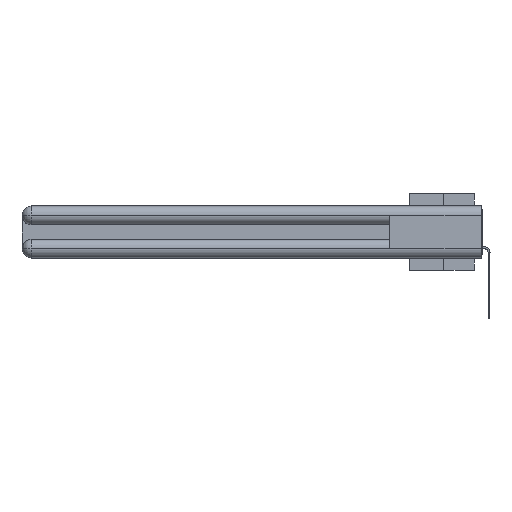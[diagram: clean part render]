
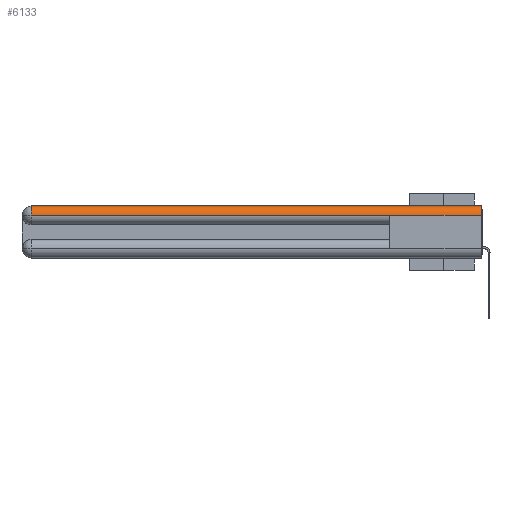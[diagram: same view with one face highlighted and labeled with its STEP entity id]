
A CAD part, left-side view. The second image highlights one B-rep face of the part: STEP entity #6133.
In plain terms, the highlighted cylindrical face has radius 1.562 mm (diameter 3.124 mm), a partial arc.
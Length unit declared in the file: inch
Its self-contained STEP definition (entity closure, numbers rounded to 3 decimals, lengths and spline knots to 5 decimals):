
#640 = VERTEX_POINT ( 'NONE', #28494 ) ;
#670 = VERTEX_POINT ( 'NONE', #4784 ) ;
#1827 = ORIENTED_EDGE ( 'NONE', *, *, #25574, .F. ) ;
#1966 = CARTESIAN_POINT ( 'NONE',  ( 0.0615, 2.94, -0.0615 ) ) ;
#2603 = DIRECTION ( 'NONE',  ( 0., -1., 0. ) ) ;
#3129 = CIRCLE ( 'NONE', #20891, 0.0615 ) ;
#4360 = DIRECTION ( 'NONE',  ( 0., 0., 1. ) ) ;
#4784 = CARTESIAN_POINT ( 'NONE',  ( 0.0615, 0., 0. ) ) ;
#6133 = ADVANCED_FACE ( 'NONE', ( #8679 ), #9038, .T. ) ;
#7046 = VERTEX_POINT ( 'NONE', #27133 ) ;
#7271 = DIRECTION ( 'NONE',  ( 1., 0., 0. ) ) ;
#7306 = DIRECTION ( 'NONE',  ( 0., -1., 0. ) ) ;
#8679 = FACE_OUTER_BOUND ( 'NONE', #14343, .T. ) ;
#9038 = CYLINDRICAL_SURFACE ( 'NONE', #29739, 0.0615 ) ;
#9051 = LINE ( 'NONE', #30841, #21299 ) ;
#9223 = LINE ( 'NONE', #12242, #25432 ) ;
#11766 = DIRECTION ( 'NONE',  ( 0., 1., 0. ) ) ;
#11926 = ORIENTED_EDGE ( 'NONE', *, *, #16208, .T. ) ;
#11950 = EDGE_CURVE ( 'NONE', #670, #27928, #26393, .T. ) ;
#12242 = CARTESIAN_POINT ( 'NONE',  ( 0., 3., -0.0615 ) ) ;
#13227 = EDGE_CURVE ( 'NONE', #27928, #7046, #9223, .T. ) ;
#13975 = DIRECTION ( 'NONE',  ( 0., 0., 1. ) ) ;
#14343 = EDGE_LOOP ( 'NONE', ( #1827, #11926, #28306, #26426, #21880 ) ) ;
#16208 = EDGE_CURVE ( 'NONE', #22157, #640, #3129, .T. ) ;
#16525 = DIRECTION ( 'NONE',  ( 0., 1., 0. ) ) ;
#16729 = VECTOR ( 'NONE', #21988, 39.37008 ) ;
#16813 = CARTESIAN_POINT ( 'NONE',  ( 0.0615, 0., -0.0615 ) ) ;
#17289 = DIRECTION ( 'NONE',  ( 0., -1., 0. ) ) ;
#20286 = AXIS2_PLACEMENT_3D ( 'NONE', #16813, #17289, #7271 ) ;
#20891 = AXIS2_PLACEMENT_3D ( 'NONE', #1966, #2603, #4360 ) ;
#21299 = VECTOR ( 'NONE', #7306, 39.37008 ) ;
#21880 = ORIENTED_EDGE ( 'NONE', *, *, #11950, .F. ) ;
#21988 = DIRECTION ( 'NONE',  ( 0., -1., 0. ) ) ;
#22157 = VERTEX_POINT ( 'NONE', #23263 ) ;
#23263 = CARTESIAN_POINT ( 'NONE',  ( 0.0615, 2.94, 0. ) ) ;
#24323 = CARTESIAN_POINT ( 'NONE',  ( 0., 0., -0.0615 ) ) ;
#24378 = LINE ( 'NONE', #29320, #16729 ) ;
#25432 = VECTOR ( 'NONE', #16525, 39.37008 ) ;
#25574 = EDGE_CURVE ( 'NONE', #22157, #670, #9051, .T. ) ;
#26393 = CIRCLE ( 'NONE', #20286, 0.0615 ) ;
#26426 = ORIENTED_EDGE ( 'NONE', *, *, #13227, .F. ) ;
#27133 = CARTESIAN_POINT ( 'NONE',  ( 0., 0.6, -0.0615 ) ) ;
#27928 = VERTEX_POINT ( 'NONE', #24323 ) ;
#28306 = ORIENTED_EDGE ( 'NONE', *, *, #30579, .T. ) ;
#28494 = CARTESIAN_POINT ( 'NONE',  ( 0., 2.94, -0.0615 ) ) ;
#29320 = CARTESIAN_POINT ( 'NONE',  ( 0., 3., -0.0615 ) ) ;
#29739 = AXIS2_PLACEMENT_3D ( 'NONE', #31309, #11766, #13975 ) ;
#30579 = EDGE_CURVE ( 'NONE', #640, #7046, #24378, .T. ) ;
#30841 = CARTESIAN_POINT ( 'NONE',  ( 0.0615, 0., 0. ) ) ;
#31309 = CARTESIAN_POINT ( 'NONE',  ( 0.0615, 0., -0.0615 ) ) ;
